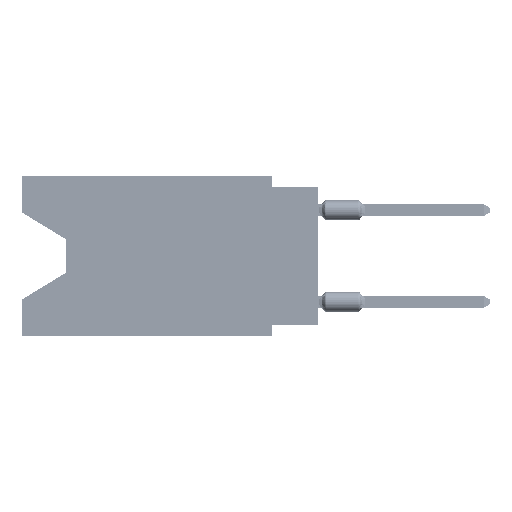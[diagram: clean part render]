
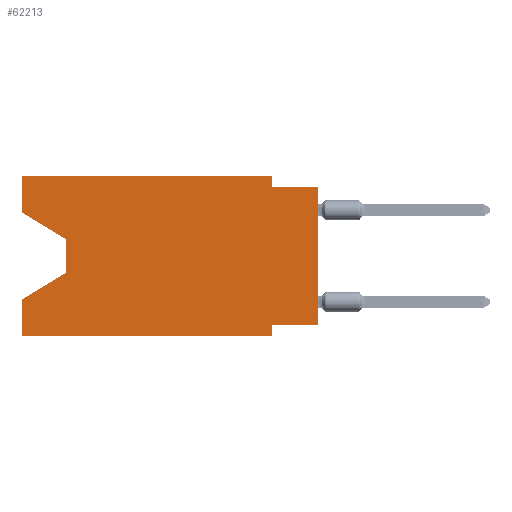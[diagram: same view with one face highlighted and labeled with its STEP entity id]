
A CAD part, left-side view. The second image highlights one B-rep face of the part: STEP entity #62213.
In plain terms, the highlighted planar face has unit normal (-1, 0, 0).
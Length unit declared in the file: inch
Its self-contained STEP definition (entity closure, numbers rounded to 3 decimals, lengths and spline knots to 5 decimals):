
#38 = CARTESIAN_POINT ( 'NONE',  ( 0., 0.55, -0.138 ) ) ;
#564 = CARTESIAN_POINT ( 'NONE',  ( 0., 0.645, -0.35 ) ) ;
#1979 = CARTESIAN_POINT ( 'NONE',  ( 0., 0.645, -0.26975 ) ) ;
#2738 = DIRECTION ( 'NONE',  ( 0., 0., 1. ) ) ;
#2861 = VECTOR ( 'NONE', #58977, 39.37008 ) ;
#3105 = LINE ( 'NONE', #41732, #15760 ) ;
#3497 = CARTESIAN_POINT ( 'NONE',  ( 0., 0.645, 0. ) ) ;
#3798 = EDGE_CURVE ( 'NONE', #59147, #32201, #17946, .T. ) ;
#4547 = LINE ( 'NONE', #31726, #14715 ) ;
#5112 = PLANE ( 'NONE',  #52244 ) ;
#7947 = ORIENTED_EDGE ( 'NONE', *, *, #27222, .T. ) ;
#8740 = CARTESIAN_POINT ( 'NONE',  ( 0., 0.1, 0. ) ) ;
#8869 = VECTOR ( 'NONE', #38870, 39.37008 ) ;
#9102 = LINE ( 'NONE', #8740, #37514 ) ;
#9108 = VECTOR ( 'NONE', #11815, 39.37008 ) ;
#9425 = ORIENTED_EDGE ( 'NONE', *, *, #58798, .F. ) ;
#9427 = DIRECTION ( 'NONE',  ( 1., 0., 0. ) ) ;
#9537 = EDGE_CURVE ( 'NONE', #27686, #11496, #37483, .T. ) ;
#9844 = CARTESIAN_POINT ( 'NONE',  ( 0., 0., 0. ) ) ;
#10212 = LINE ( 'NONE', #9844, #13092 ) ;
#10715 = ORIENTED_EDGE ( 'NONE', *, *, #66939, .T. ) ;
#11410 = CARTESIAN_POINT ( 'NONE',  ( 0., 0.1, -0.025 ) ) ;
#11496 = VERTEX_POINT ( 'NONE', #23323 ) ;
#11815 = DIRECTION ( 'NONE',  ( 0., 0.855, -0.519 ) ) ;
#13092 = VECTOR ( 'NONE', #64633, 39.37008 ) ;
#14563 = DIRECTION ( 'NONE',  ( 0., 0., -1. ) ) ;
#14715 = VECTOR ( 'NONE', #37453, 39.37008 ) ;
#15760 = VECTOR ( 'NONE', #14563, 39.37008 ) ;
#17392 = ORIENTED_EDGE ( 'NONE', *, *, #47681, .F. ) ;
#17743 = CARTESIAN_POINT ( 'NONE',  ( 0., 0.55, -0.138 ) ) ;
#17946 = LINE ( 'NONE', #65941, #46987 ) ;
#18592 = CARTESIAN_POINT ( 'NONE',  ( 0., 0., -0.325 ) ) ;
#18642 = CARTESIAN_POINT ( 'NONE',  ( 0., 0.55, -0.212 ) ) ;
#19742 = EDGE_CURVE ( 'NONE', #51462, #32783, #4547, .T. ) ;
#20971 = EDGE_CURVE ( 'NONE', #57726, #55810, #64701, .T. ) ;
#21057 = EDGE_CURVE ( 'NONE', #56333, #57726, #30679, .T. ) ;
#21225 = CARTESIAN_POINT ( 'NONE',  ( 0., 0.645, 0. ) ) ;
#21389 = CARTESIAN_POINT ( 'NONE',  ( 0., 0., -0.325 ) ) ;
#21751 = VECTOR ( 'NONE', #43212, 39.37008 ) ;
#22974 = ORIENTED_EDGE ( 'NONE', *, *, #9537, .F. ) ;
#23323 = CARTESIAN_POINT ( 'NONE',  ( 0., 0.1, -0.325 ) ) ;
#25324 = DIRECTION ( 'NONE',  ( 0., 0., 1. ) ) ;
#27222 = EDGE_CURVE ( 'NONE', #27686, #32783, #10212, .T. ) ;
#27686 = VERTEX_POINT ( 'NONE', #18592 ) ;
#30552 = DIRECTION ( 'NONE',  ( 0., 0., -1. ) ) ;
#30631 = CARTESIAN_POINT ( 'NONE',  ( 0., 0.1, 0. ) ) ;
#30679 = LINE ( 'NONE', #3497, #65780 ) ;
#31726 = CARTESIAN_POINT ( 'NONE',  ( 0., 0., -0.025 ) ) ;
#32201 = VERTEX_POINT ( 'NONE', #34039 ) ;
#32783 = VERTEX_POINT ( 'NONE', #40361 ) ;
#33290 = LINE ( 'NONE', #39008, #9108 ) ;
#34039 = CARTESIAN_POINT ( 'NONE',  ( 0., 0.1, -0.35 ) ) ;
#35993 = VECTOR ( 'NONE', #61236, 39.37008 ) ;
#36283 = CARTESIAN_POINT ( 'NONE',  ( 0., 0.645, -0.08025 ) ) ;
#37026 = ORIENTED_EDGE ( 'NONE', *, *, #20971, .F. ) ;
#37453 = DIRECTION ( 'NONE',  ( 0., -1., 0. ) ) ;
#37483 = LINE ( 'NONE', #21389, #21751 ) ;
#37514 = VECTOR ( 'NONE', #30552, 39.37008 ) ;
#38870 = DIRECTION ( 'NONE',  ( 0., 0., -1. ) ) ;
#39008 = CARTESIAN_POINT ( 'NONE',  ( 0., 0.55, -0.212 ) ) ;
#39362 = CARTESIAN_POINT ( 'NONE',  ( 0., 0.645, -0.08025 ) ) ;
#39868 = VECTOR ( 'NONE', #2738, 39.37008 ) ;
#40361 = CARTESIAN_POINT ( 'NONE',  ( 0., 0., -0.025 ) ) ;
#40379 = VERTEX_POINT ( 'NONE', #18642 ) ;
#41112 = EDGE_LOOP ( 'NONE', ( #69159, #41165, #10715, #41412, #69856, #9425, #22974, #7947, #42166, #17392, #37026, #70753 ) ) ;
#41165 = ORIENTED_EDGE ( 'NONE', *, *, #44989, .T. ) ;
#41412 = ORIENTED_EDGE ( 'NONE', *, *, #61741, .F. ) ;
#41732 = CARTESIAN_POINT ( 'NONE',  ( 0., 0.1, -0.35 ) ) ;
#41872 = EDGE_CURVE ( 'NONE', #56333, #42918, #66259, .T. ) ;
#42166 = ORIENTED_EDGE ( 'NONE', *, *, #19742, .F. ) ;
#42918 = VERTEX_POINT ( 'NONE', #38 ) ;
#43212 = DIRECTION ( 'NONE',  ( 0., 1., 0. ) ) ;
#44464 = DIRECTION ( 'NONE',  ( 0., -1., 0. ) ) ;
#44989 = EDGE_CURVE ( 'NONE', #42918, #40379, #66454, .T. ) ;
#46987 = VECTOR ( 'NONE', #44464, 39.37008 ) ;
#47482 = VERTEX_POINT ( 'NONE', #1979 ) ;
#47681 = EDGE_CURVE ( 'NONE', #55810, #51462, #9102, .T. ) ;
#47720 = DIRECTION ( 'NONE',  ( 0., 0., -1. ) ) ;
#51462 = VERTEX_POINT ( 'NONE', #11410 ) ;
#52244 = AXIS2_PLACEMENT_3D ( 'NONE', #59190, #9427, #47720 ) ;
#55810 = VERTEX_POINT ( 'NONE', #30631 ) ;
#56333 = VERTEX_POINT ( 'NONE', #36283 ) ;
#57726 = VERTEX_POINT ( 'NONE', #21225 ) ;
#58798 = EDGE_CURVE ( 'NONE', #11496, #32201, #3105, .T. ) ;
#58977 = DIRECTION ( 'NONE',  ( 0., -1., 0. ) ) ;
#59147 = VERTEX_POINT ( 'NONE', #564 ) ;
#59190 = CARTESIAN_POINT ( 'NONE',  ( 0., 0.645, 0. ) ) ;
#59546 = FACE_OUTER_BOUND ( 'NONE', #41112, .T. ) ;
#61236 = DIRECTION ( 'NONE',  ( 0., -0.855, -0.519 ) ) ;
#61741 = EDGE_CURVE ( 'NONE', #59147, #47482, #62893, .T. ) ;
#62213 = ADVANCED_FACE ( 'NONE', ( #59546 ), #5112, .F. ) ;
#62893 = LINE ( 'NONE', #63953, #39868 ) ;
#63953 = CARTESIAN_POINT ( 'NONE',  ( 0., 0.645, 0. ) ) ;
#64633 = DIRECTION ( 'NONE',  ( 0., 0., 1. ) ) ;
#64701 = LINE ( 'NONE', #68984, #2861 ) ;
#65780 = VECTOR ( 'NONE', #25324, 39.37008 ) ;
#65941 = CARTESIAN_POINT ( 'NONE',  ( 0., 0.645, -0.35 ) ) ;
#66259 = LINE ( 'NONE', #39362, #35993 ) ;
#66454 = LINE ( 'NONE', #17743, #8869 ) ;
#66939 = EDGE_CURVE ( 'NONE', #40379, #47482, #33290, .T. ) ;
#68984 = CARTESIAN_POINT ( 'NONE',  ( 0., 0.645, 0. ) ) ;
#69159 = ORIENTED_EDGE ( 'NONE', *, *, #41872, .T. ) ;
#69856 = ORIENTED_EDGE ( 'NONE', *, *, #3798, .T. ) ;
#70753 = ORIENTED_EDGE ( 'NONE', *, *, #21057, .F. ) ;
